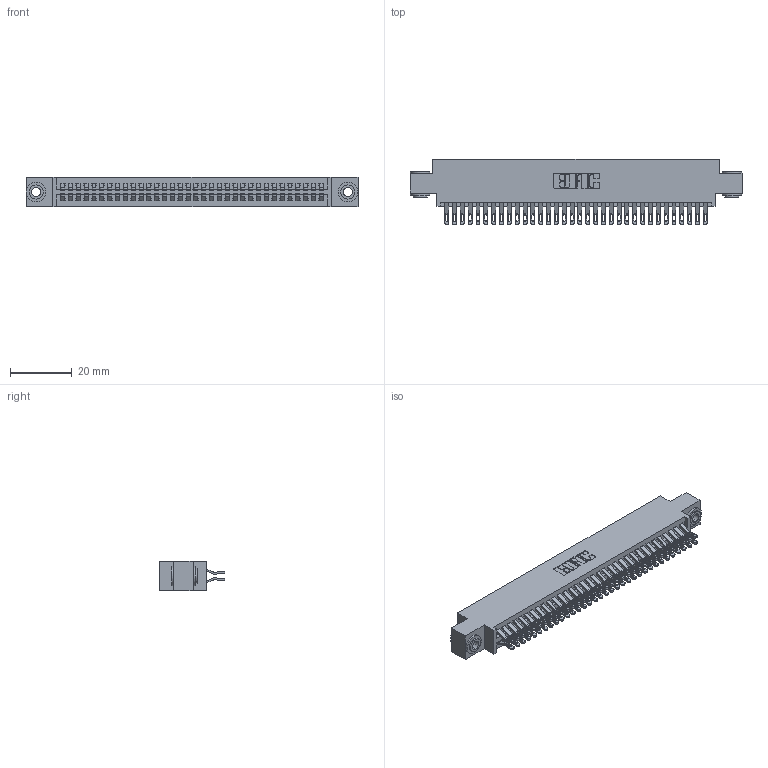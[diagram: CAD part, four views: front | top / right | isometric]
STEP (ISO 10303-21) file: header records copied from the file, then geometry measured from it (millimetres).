
FILE_DESCRIPTION (( 'STEP AP203' ), '1' );
FILE_NAME ('345-068-555-803.STEP', '2018-09-30T14:21:45', ( '' ), ( '' ), 'SwSTEP 2.0', 'SolidWorks 2016', '' );
FILE_SCHEMA (( 'CONFIG_CONTROL_DESIGN' ));
Length unit declared in the file: inch
Products named in the file (4): 345 Part_0.170 Offset - 0.156 Dia-TH; 345-292-001_555 Tail; 345-250-002_345-250-002-102; 345-068-555-803
Assembly tree (71 placements, depth 2):
  345-068-555-803
    345 Part_0.170 Offset - 0.156 Dia-TH
    345-292-001_555 Tail  x68
    345-250-002_345-250-002-102  x2
Bounding box: 107.57 x 21.13 x 9.4 mm (x, y, z)
Volume: 10478.4 mm3; surface area: 16368.2 mm2
Topology: 71 solids, 71 shells, 3976 faces, 12465 edges, 8306 vertices
Faces by surface type: plane 2202, cylinder 1766, cone 8
Entity records: 28862 total; most frequent: CARTESIAN_POINT 4857, ORIENTED_EDGE 4754, DIRECTION 4291, EDGE_CURVE 2377, VECTOR 2065, LINE 2065, VERTEX_POINT 1582, AXIS2_PLACEMENT_3D 1113
